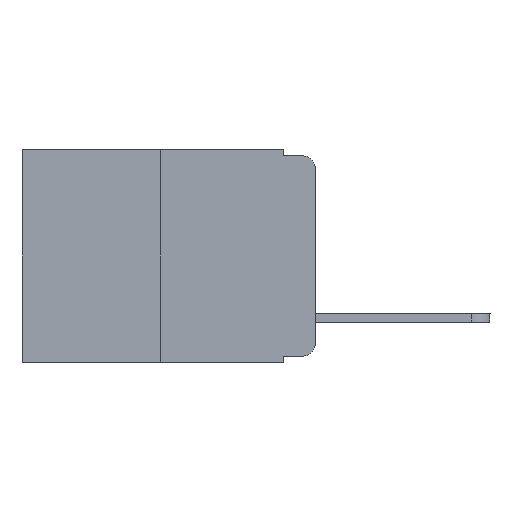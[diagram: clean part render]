
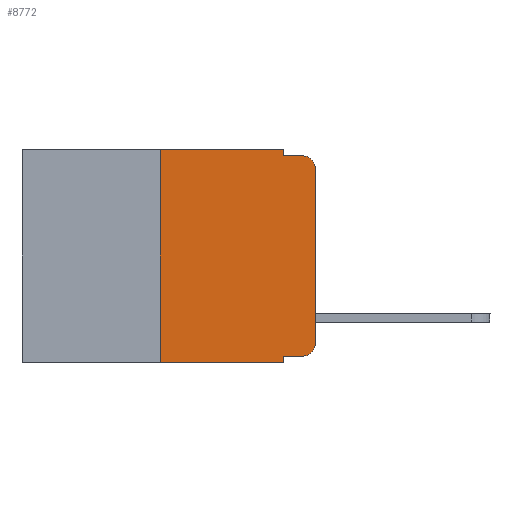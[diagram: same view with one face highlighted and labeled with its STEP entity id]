
A CAD part, left-side view. The second image highlights one B-rep face of the part: STEP entity #8772.
In plain terms, the highlighted planar face has unit normal (-1, 0, 0).
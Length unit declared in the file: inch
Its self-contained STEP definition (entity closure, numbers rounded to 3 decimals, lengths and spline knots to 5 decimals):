
#197 = EDGE_CURVE ( 'NONE', #23703, #7690, #17532, .T. ) ;
#223 = EDGE_CURVE ( 'NONE', #4554, #6653, #19249, .T. ) ;
#299 = CARTESIAN_POINT ( 'NONE',  ( 0., 0.02, -0.03 ) ) ;
#302 = DIRECTION ( 'NONE',  ( 0., 0., -1. ) ) ;
#552 = ORIENTED_EDGE ( 'NONE', *, *, #8871, .F. ) ;
#704 = DIRECTION ( 'NONE',  ( 0., 0., -1. ) ) ;
#1055 = ORIENTED_EDGE ( 'NONE', *, *, #3168, .T. ) ;
#1883 = AXIS2_PLACEMENT_3D ( 'NONE', #4144, #22522, #302 ) ;
#1900 = VECTOR ( 'NONE', #7640, 39.37008 ) ;
#1993 = VERTEX_POINT ( 'NONE', #17283 ) ;
#2259 = VECTOR ( 'NONE', #704, 39.37008 ) ;
#2555 = DIRECTION ( 'NONE',  ( -1., 0., 0. ) ) ;
#2658 = ORIENTED_EDGE ( 'NONE', *, *, #23285, .F. ) ;
#3168 = EDGE_CURVE ( 'NONE', #13476, #23703, #16655, .T. ) ;
#3668 = VECTOR ( 'NONE', #6923, 39.37008 ) ;
#4144 = CARTESIAN_POINT ( 'NONE',  ( 0., 0.473, 0. ) ) ;
#4554 = VERTEX_POINT ( 'NONE', #10078 ) ;
#4842 = VECTOR ( 'NONE', #25278, 39.37008 ) ;
#5012 = VECTOR ( 'NONE', #18806, 39.37008 ) ;
#5648 = CARTESIAN_POINT ( 'NONE',  ( 0., 0., -0.313 ) ) ;
#5805 = LINE ( 'NONE', #11517, #19815 ) ;
#6124 = ORIENTED_EDGE ( 'NONE', *, *, #23616, .T. ) ;
#6210 = CARTESIAN_POINT ( 'NONE',  ( 0., 0.051, -0.343 ) ) ;
#6653 = VERTEX_POINT ( 'NONE', #22179 ) ;
#6923 = DIRECTION ( 'NONE',  ( 0., 0., 1. ) ) ;
#7202 = EDGE_CURVE ( 'NONE', #1993, #22211, #24654, .T. ) ;
#7640 = DIRECTION ( 'NONE',  ( 0., -1., 0. ) ) ;
#7690 = VERTEX_POINT ( 'NONE', #16481 ) ;
#8255 = DIRECTION ( 'NONE',  ( -1., 0., 0. ) ) ;
#8352 = CARTESIAN_POINT ( 'NONE',  ( 0., 0.473, 0. ) ) ;
#8394 = DIRECTION ( 'NONE',  ( 0., 0., -1. ) ) ;
#8613 = AXIS2_PLACEMENT_3D ( 'NONE', #17023, #2555, #21096 ) ;
#8626 = ORIENTED_EDGE ( 'NONE', *, *, #13417, .T. ) ;
#8772 = ADVANCED_FACE ( 'NONE', ( #22393 ), #12611, .F. ) ;
#8871 = EDGE_CURVE ( 'NONE', #18183, #20882, #15142, .T. ) ;
#9757 = LINE ( 'NONE', #17866, #1900 ) ;
#10078 = CARTESIAN_POINT ( 'NONE',  ( 0., 0.25, -0.343 ) ) ;
#10719 = CARTESIAN_POINT ( 'NONE',  ( 0., 0.051, -0.01 ) ) ;
#11467 = ORIENTED_EDGE ( 'NONE', *, *, #16208, .T. ) ;
#11517 = CARTESIAN_POINT ( 'NONE',  ( 0., 0.051, -0.333 ) ) ;
#12611 = PLANE ( 'NONE',  #1883 ) ;
#12982 = CARTESIAN_POINT ( 'NONE',  ( 0., 0.051, 0. ) ) ;
#13144 = DIRECTION ( 'NONE',  ( 0., 0., 1. ) ) ;
#13417 = EDGE_CURVE ( 'NONE', #1993, #13476, #5805, .T. ) ;
#13454 = ORIENTED_EDGE ( 'NONE', *, *, #7202, .F. ) ;
#13476 = VERTEX_POINT ( 'NONE', #23535 ) ;
#13591 = ORIENTED_EDGE ( 'NONE', *, *, #223, .F. ) ;
#14830 = DIRECTION ( 'NONE',  ( 0., -1., 0. ) ) ;
#14963 = EDGE_CURVE ( 'NONE', #20882, #23172, #17087, .T. ) ;
#15142 = LINE ( 'NONE', #19106, #4842 ) ;
#16208 = EDGE_CURVE ( 'NONE', #7690, #23172, #22374, .T. ) ;
#16481 = CARTESIAN_POINT ( 'NONE',  ( 0., 0., -0.03 ) ) ;
#16655 = CIRCLE ( 'NONE', #8613, 0.02 ) ;
#16769 = CARTESIAN_POINT ( 'NONE',  ( 0., 0.051, 0. ) ) ;
#17023 = CARTESIAN_POINT ( 'NONE',  ( 0., 0.02, -0.313 ) ) ;
#17087 = LINE ( 'NONE', #10719, #5012 ) ;
#17283 = CARTESIAN_POINT ( 'NONE',  ( 0., 0.051, -0.333 ) ) ;
#17532 = LINE ( 'NONE', #21333, #17646 ) ;
#17646 = VECTOR ( 'NONE', #13144, 39.37008 ) ;
#17748 = EDGE_LOOP ( 'NONE', ( #24832, #11467, #21600, #552, #2658, #13591, #6124, #13454, #8626, #1055 ) ) ;
#17866 = CARTESIAN_POINT ( 'NONE',  ( 0., 0.473, -0.343 ) ) ;
#18178 = CARTESIAN_POINT ( 'NONE',  ( 0., 0.02, -0.01 ) ) ;
#18183 = VERTEX_POINT ( 'NONE', #12982 ) ;
#18806 = DIRECTION ( 'NONE',  ( 0., -1., 0. ) ) ;
#19106 = CARTESIAN_POINT ( 'NONE',  ( 0., 0.051, 0. ) ) ;
#19249 = LINE ( 'NONE', #25023, #3668 ) ;
#19815 = VECTOR ( 'NONE', #21950, 39.37008 ) ;
#20557 = VECTOR ( 'NONE', #14830, 39.37008 ) ;
#20882 = VERTEX_POINT ( 'NONE', #26171 ) ;
#21096 = DIRECTION ( 'NONE',  ( 0., 0., -1. ) ) ;
#21333 = CARTESIAN_POINT ( 'NONE',  ( 0., 0., 0. ) ) ;
#21600 = ORIENTED_EDGE ( 'NONE', *, *, #14963, .F. ) ;
#21950 = DIRECTION ( 'NONE',  ( 0., -1., 0. ) ) ;
#22179 = CARTESIAN_POINT ( 'NONE',  ( 0., 0.25, 0. ) ) ;
#22211 = VERTEX_POINT ( 'NONE', #6210 ) ;
#22374 = CIRCLE ( 'NONE', #23664, 0.02 ) ;
#22393 = FACE_OUTER_BOUND ( 'NONE', #17748, .T. ) ;
#22522 = DIRECTION ( 'NONE',  ( 1., 0., 0. ) ) ;
#23172 = VERTEX_POINT ( 'NONE', #18178 ) ;
#23285 = EDGE_CURVE ( 'NONE', #6653, #18183, #24335, .T. ) ;
#23535 = CARTESIAN_POINT ( 'NONE',  ( 0., 0.02, -0.333 ) ) ;
#23616 = EDGE_CURVE ( 'NONE', #4554, #22211, #9757, .T. ) ;
#23664 = AXIS2_PLACEMENT_3D ( 'NONE', #299, #8255, #8394 ) ;
#23703 = VERTEX_POINT ( 'NONE', #5648 ) ;
#24335 = LINE ( 'NONE', #8352, #20557 ) ;
#24654 = LINE ( 'NONE', #16769, #2259 ) ;
#24832 = ORIENTED_EDGE ( 'NONE', *, *, #197, .T. ) ;
#25023 = CARTESIAN_POINT ( 'NONE',  ( 0., 0.25, 0. ) ) ;
#25278 = DIRECTION ( 'NONE',  ( 0., 0., -1. ) ) ;
#26171 = CARTESIAN_POINT ( 'NONE',  ( 0., 0.051, -0.01 ) ) ;
